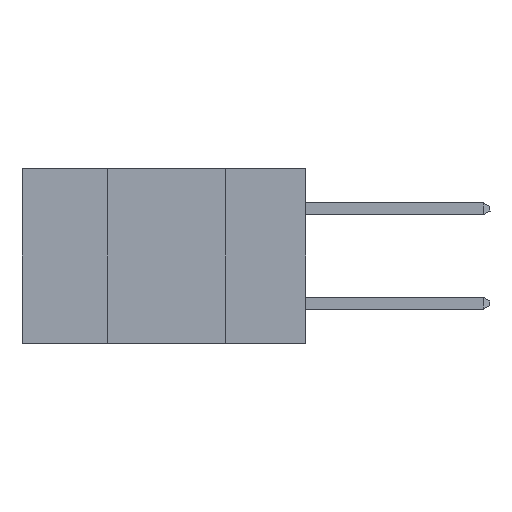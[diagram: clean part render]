
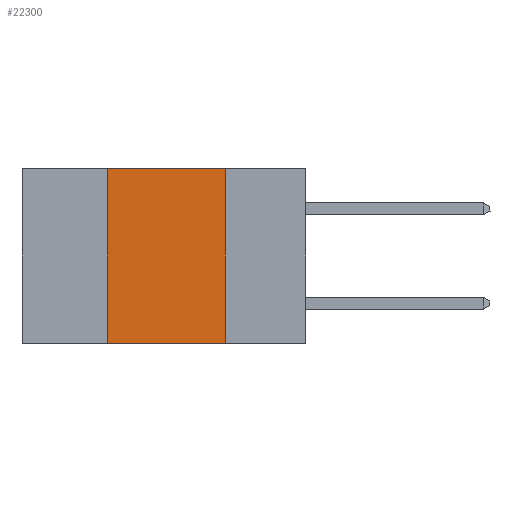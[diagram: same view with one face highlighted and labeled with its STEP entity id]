
A CAD part, left-side view. The second image highlights one B-rep face of the part: STEP entity #22300.
In plain terms, the highlighted planar face has unit normal (-1, 0, 0).
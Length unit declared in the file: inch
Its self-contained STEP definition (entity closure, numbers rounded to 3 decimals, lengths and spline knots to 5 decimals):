
#280 = CARTESIAN_POINT ( 'NONE',  ( 0., 0.17, 0. ) ) ;
#2460 = EDGE_CURVE ( 'NONE', #26814, #12893, #11878, .T. ) ;
#2688 = PLANE ( 'NONE',  #22564 ) ;
#3483 = ORIENTED_EDGE ( 'NONE', *, *, #21204, .F. ) ;
#3575 = CARTESIAN_POINT ( 'NONE',  ( 0., 0.17, 0. ) ) ;
#3736 = DIRECTION ( 'NONE',  ( 1., 0., 0. ) ) ;
#4822 = ORIENTED_EDGE ( 'NONE', *, *, #2460, .F. ) ;
#6361 = VERTEX_POINT ( 'NONE', #19185 ) ;
#6445 = CARTESIAN_POINT ( 'NONE',  ( 0., 0.17, -0.37 ) ) ;
#7881 = VERTEX_POINT ( 'NONE', #6445 ) ;
#10752 = VECTOR ( 'NONE', #11912, 39.37008 ) ;
#11051 = DIRECTION ( 'NONE',  ( 0., 0., 1. ) ) ;
#11595 = ORIENTED_EDGE ( 'NONE', *, *, #17046, .F. ) ;
#11855 = EDGE_LOOP ( 'NONE', ( #3483, #4822, #11595, #22589 ) ) ;
#11878 = LINE ( 'NONE', #18773, #22880 ) ;
#11912 = DIRECTION ( 'NONE',  ( 0., 0., -1. ) ) ;
#12893 = VERTEX_POINT ( 'NONE', #280 ) ;
#13437 = VECTOR ( 'NONE', #11051, 39.37008 ) ;
#13992 = DIRECTION ( 'NONE',  ( 0., -1., 0. ) ) ;
#15150 = CARTESIAN_POINT ( 'NONE',  ( 0., 0.6, 0. ) ) ;
#15497 = VECTOR ( 'NONE', #16468, 39.37008 ) ;
#15660 = EDGE_CURVE ( 'NONE', #6361, #7881, #26307, .T. ) ;
#16226 = LINE ( 'NONE', #3575, #10752 ) ;
#16468 = DIRECTION ( 'NONE',  ( 0., -1., 0. ) ) ;
#17046 = EDGE_CURVE ( 'NONE', #6361, #26814, #18956, .T. ) ;
#17050 = FACE_OUTER_BOUND ( 'NONE', #11855, .T. ) ;
#18114 = DIRECTION ( 'NONE',  ( 0., 0., -1. ) ) ;
#18773 = CARTESIAN_POINT ( 'NONE',  ( 0., 0.6, 0. ) ) ;
#18956 = LINE ( 'NONE', #25386, #13437 ) ;
#19185 = CARTESIAN_POINT ( 'NONE',  ( 0., 0.42, -0.37 ) ) ;
#20188 = CARTESIAN_POINT ( 'NONE',  ( 0., 0.42, 0. ) ) ;
#21204 = EDGE_CURVE ( 'NONE', #12893, #7881, #16226, .T. ) ;
#22300 = ADVANCED_FACE ( 'NONE', ( #17050 ), #2688, .F. ) ;
#22564 = AXIS2_PLACEMENT_3D ( 'NONE', #15150, #3736, #18114 ) ;
#22589 = ORIENTED_EDGE ( 'NONE', *, *, #15660, .T. ) ;
#22880 = VECTOR ( 'NONE', #13992, 39.37008 ) ;
#25386 = CARTESIAN_POINT ( 'NONE',  ( 0., 0.42, 0. ) ) ;
#26307 = LINE ( 'NONE', #26614, #15497 ) ;
#26614 = CARTESIAN_POINT ( 'NONE',  ( 0., 0.6, -0.37 ) ) ;
#26814 = VERTEX_POINT ( 'NONE', #20188 ) ;
